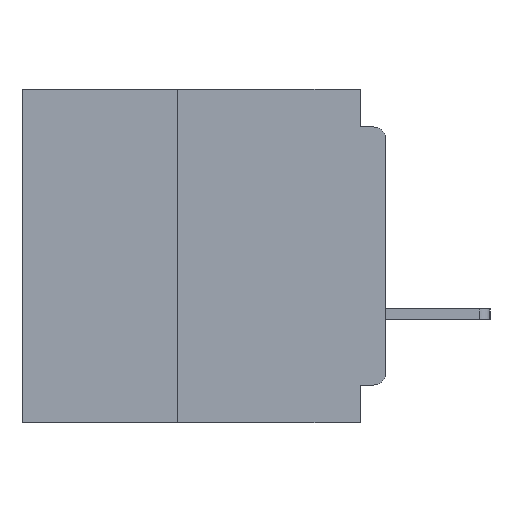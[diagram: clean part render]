
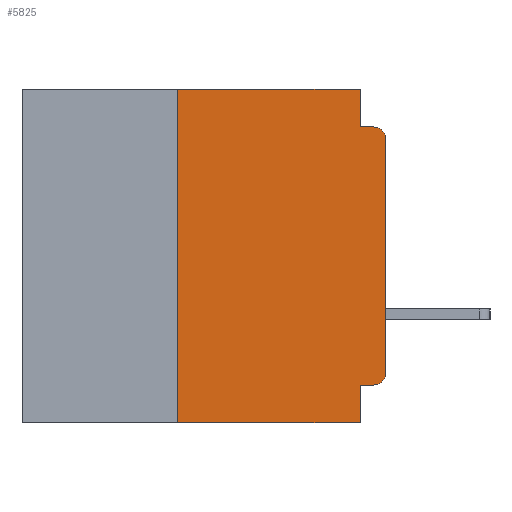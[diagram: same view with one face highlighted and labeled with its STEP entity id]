
A CAD part, left-side view. The second image highlights one B-rep face of the part: STEP entity #5825.
In plain terms, the highlighted planar face has unit normal (-1, 0, 0).
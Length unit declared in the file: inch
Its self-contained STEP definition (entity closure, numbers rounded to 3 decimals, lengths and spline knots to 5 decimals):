
#1058 = VERTEX_POINT ( 'NONE', #54549 ) ;
#1269 = AXIS2_PLACEMENT_3D ( 'NONE', #60084, #2671, #36244 ) ;
#2659 = EDGE_CURVE ( 'NONE', #4595, #14468, #49981, .T. ) ;
#2671 = DIRECTION ( 'NONE',  ( 1., 0., 0. ) ) ;
#3395 = VECTOR ( 'NONE', #31444, 39.37008 ) ;
#4595 = VERTEX_POINT ( 'NONE', #31244 ) ;
#4651 = EDGE_CURVE ( 'NONE', #34081, #1058, #22165, .T. ) ;
#4983 = CARTESIAN_POINT ( 'NONE',  ( 0., 0., -0.34 ) ) ;
#5623 = VERTEX_POINT ( 'NONE', #24919 ) ;
#5825 = ADVANCED_FACE ( 'NONE', ( #9197 ), #55449, .F. ) ;
#5830 = CARTESIAN_POINT ( 'NONE',  ( 0., 0., -0.045 ) ) ;
#6897 = DIRECTION ( 'NONE',  ( -1., 0., 0. ) ) ;
#7336 = EDGE_CURVE ( 'NONE', #46172, #34081, #9744, .T. ) ;
#8621 = ORIENTED_EDGE ( 'NONE', *, *, #49734, .T. ) ;
#9197 = FACE_OUTER_BOUND ( 'NONE', #62439, .T. ) ;
#9744 = LINE ( 'NONE', #10629, #22524 ) ;
#9966 = VECTOR ( 'NONE', #52173, 39.37008 ) ;
#10629 = CARTESIAN_POINT ( 'NONE',  ( 0., 0.25, -0.4 ) ) ;
#11875 = CARTESIAN_POINT ( 'NONE',  ( 0., 0.437, -0.4 ) ) ;
#12779 = CARTESIAN_POINT ( 'NONE',  ( 0., 0., 0. ) ) ;
#12885 = ORIENTED_EDGE ( 'NONE', *, *, #7336, .F. ) ;
#13506 = CARTESIAN_POINT ( 'NONE',  ( 0., 0.015, -0.34 ) ) ;
#14468 = VERTEX_POINT ( 'NONE', #48987 ) ;
#15067 = ORIENTED_EDGE ( 'NONE', *, *, #27056, .T. ) ;
#15466 = CARTESIAN_POINT ( 'NONE',  ( 0., 0., -0.355 ) ) ;
#16555 = EDGE_CURVE ( 'NONE', #26372, #5623, #22153, .T. ) ;
#16703 = DIRECTION ( 'NONE',  ( 0., -1., 0. ) ) ;
#17615 = EDGE_CURVE ( 'NONE', #1058, #26372, #48325, .T. ) ;
#18338 = DIRECTION ( 'NONE',  ( 0., 0., -1. ) ) ;
#18478 = ORIENTED_EDGE ( 'NONE', *, *, #31532, .T. ) ;
#18517 = CARTESIAN_POINT ( 'NONE',  ( 0., 0.031, -0.4 ) ) ;
#19068 = VERTEX_POINT ( 'NONE', #62401 ) ;
#19094 = VECTOR ( 'NONE', #61475, 39.37008 ) ;
#22153 = LINE ( 'NONE', #5830, #60585 ) ;
#22165 = LINE ( 'NONE', #50611, #3395 ) ;
#22524 = VECTOR ( 'NONE', #29790, 39.37008 ) ;
#23139 = LINE ( 'NONE', #11875, #60079 ) ;
#24719 = VERTEX_POINT ( 'NONE', #18517 ) ;
#24919 = CARTESIAN_POINT ( 'NONE',  ( 0., 0.015, -0.045 ) ) ;
#26372 = VERTEX_POINT ( 'NONE', #40807 ) ;
#27056 = EDGE_CURVE ( 'NONE', #51853, #19068, #44125, .T. ) ;
#28628 = ORIENTED_EDGE ( 'NONE', *, *, #44265, .T. ) ;
#29790 = DIRECTION ( 'NONE',  ( 0., 0., 1. ) ) ;
#29972 = DIRECTION ( 'NONE',  ( 0., 1., 0. ) ) ;
#31244 = CARTESIAN_POINT ( 'NONE',  ( 0., 0.015, -0.355 ) ) ;
#31444 = DIRECTION ( 'NONE',  ( 0., -1., 0. ) ) ;
#31532 = EDGE_CURVE ( 'NONE', #19068, #5623, #61377, .T. ) ;
#31871 = LINE ( 'NONE', #41221, #19094 ) ;
#33645 = CARTESIAN_POINT ( 'NONE',  ( 0., 0.25, -0.4 ) ) ;
#34081 = VERTEX_POINT ( 'NONE', #51529 ) ;
#35627 = CARTESIAN_POINT ( 'NONE',  ( 0., 0.015, -0.06 ) ) ;
#36244 = DIRECTION ( 'NONE',  ( 0., 0., -1. ) ) ;
#38981 = DIRECTION ( 'NONE',  ( 0., -1., 0. ) ) ;
#40476 = DIRECTION ( 'NONE',  ( 0., 0., -1. ) ) ;
#40807 = CARTESIAN_POINT ( 'NONE',  ( 0., 0.031, -0.045 ) ) ;
#41221 = CARTESIAN_POINT ( 'NONE',  ( 0., 0.031, -0.4 ) ) ;
#42312 = CIRCLE ( 'NONE', #54018, 0.015 ) ;
#44125 = LINE ( 'NONE', #12779, #55496 ) ;
#44265 = EDGE_CURVE ( 'NONE', #4595, #51853, #42312, .T. ) ;
#46172 = VERTEX_POINT ( 'NONE', #33645 ) ;
#47111 = DIRECTION ( 'NONE',  ( -1., 0., 0. ) ) ;
#47233 = ORIENTED_EDGE ( 'NONE', *, *, #2659, .F. ) ;
#47253 = AXIS2_PLACEMENT_3D ( 'NONE', #35627, #6897, #40476 ) ;
#48297 = ORIENTED_EDGE ( 'NONE', *, *, #16555, .F. ) ;
#48325 = LINE ( 'NONE', #56981, #9966 ) ;
#48987 = CARTESIAN_POINT ( 'NONE',  ( 0., 0.031, -0.355 ) ) ;
#49598 = ORIENTED_EDGE ( 'NONE', *, *, #57617, .F. ) ;
#49734 = EDGE_CURVE ( 'NONE', #46172, #24719, #23139, .T. ) ;
#49981 = LINE ( 'NONE', #15466, #61311 ) ;
#50611 = CARTESIAN_POINT ( 'NONE',  ( 0., 0.437, 0. ) ) ;
#51268 = DIRECTION ( 'NONE',  ( 0., 0., 1. ) ) ;
#51529 = CARTESIAN_POINT ( 'NONE',  ( 0., 0.25, 0. ) ) ;
#51853 = VERTEX_POINT ( 'NONE', #4983 ) ;
#52173 = DIRECTION ( 'NONE',  ( 0., 0., -1. ) ) ;
#54018 = AXIS2_PLACEMENT_3D ( 'NONE', #13506, #47111, #18338 ) ;
#54549 = CARTESIAN_POINT ( 'NONE',  ( 0., 0.031, 0. ) ) ;
#55449 = PLANE ( 'NONE',  #1269 ) ;
#55496 = VECTOR ( 'NONE', #51268, 39.37008 ) ;
#56981 = CARTESIAN_POINT ( 'NONE',  ( 0., 0.031, 0. ) ) ;
#57495 = ORIENTED_EDGE ( 'NONE', *, *, #17615, .F. ) ;
#57617 = EDGE_CURVE ( 'NONE', #14468, #24719, #31871, .T. ) ;
#60079 = VECTOR ( 'NONE', #16703, 39.37008 ) ;
#60084 = CARTESIAN_POINT ( 'NONE',  ( 0., 0.437, 0. ) ) ;
#60585 = VECTOR ( 'NONE', #38981, 39.37008 ) ;
#61311 = VECTOR ( 'NONE', #29972, 39.37008 ) ;
#61377 = CIRCLE ( 'NONE', #47253, 0.015 ) ;
#61475 = DIRECTION ( 'NONE',  ( 0., 0., -1. ) ) ;
#61714 = ORIENTED_EDGE ( 'NONE', *, *, #4651, .F. ) ;
#62401 = CARTESIAN_POINT ( 'NONE',  ( 0., 0., -0.06 ) ) ;
#62439 = EDGE_LOOP ( 'NONE', ( #15067, #18478, #48297, #57495, #61714, #12885, #8621, #49598, #47233, #28628 ) ) ;
